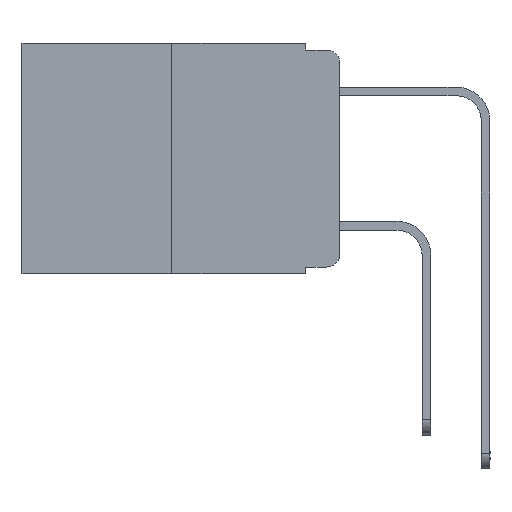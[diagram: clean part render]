
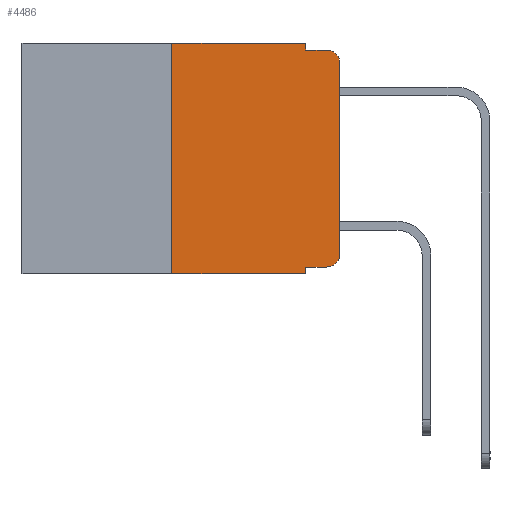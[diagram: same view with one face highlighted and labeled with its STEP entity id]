
A CAD part, left-side view. The second image highlights one B-rep face of the part: STEP entity #4486.
In plain terms, the highlighted planar face has unit normal (-1, 0, 0).
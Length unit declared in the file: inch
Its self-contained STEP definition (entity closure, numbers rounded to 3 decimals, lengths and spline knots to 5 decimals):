
#45 = DIRECTION ( 'NONE',  ( -1., 0., 0. ) ) ;
#456 = VERTEX_POINT ( 'NONE', #20318 ) ;
#701 = LINE ( 'NONE', #8829, #18971 ) ;
#1028 = VECTOR ( 'NONE', #3928, 39.37008 ) ;
#1140 = CARTESIAN_POINT ( 'NONE',  ( 0., 0.051, -0.01 ) ) ;
#1705 = DIRECTION ( 'NONE',  ( 0., 0., 1. ) ) ;
#2009 = VECTOR ( 'NONE', #10978, 39.37008 ) ;
#2176 = CARTESIAN_POINT ( 'NONE',  ( 0., 0.473, 0. ) ) ;
#2406 = LINE ( 'NONE', #10413, #20701 ) ;
#2830 = ORIENTED_EDGE ( 'NONE', *, *, #7244, .T. ) ;
#2980 = EDGE_CURVE ( 'NONE', #456, #15234, #11552, .T. ) ;
#3083 = CARTESIAN_POINT ( 'NONE',  ( 0., 0.02, -0.01 ) ) ;
#3471 = CARTESIAN_POINT ( 'NONE',  ( 0., 0.051, -0.01 ) ) ;
#3573 = CIRCLE ( 'NONE', #6258, 0.02 ) ;
#3658 = EDGE_CURVE ( 'NONE', #19618, #13431, #4326, .T. ) ;
#3928 = DIRECTION ( 'NONE',  ( 0., 0., -1. ) ) ;
#4113 = VECTOR ( 'NONE', #19249, 39.37008 ) ;
#4326 = LINE ( 'NONE', #6015, #2009 ) ;
#4486 = ADVANCED_FACE ( 'NONE', ( #10200 ), #16585, .F. ) ;
#4967 = DIRECTION ( 'NONE',  ( -1., 0., 0. ) ) ;
#5050 = DIRECTION ( 'NONE',  ( 0., -1., 0. ) ) ;
#5337 = EDGE_CURVE ( 'NONE', #8078, #17137, #15174, .T. ) ;
#5534 = CARTESIAN_POINT ( 'NONE',  ( 0., 0., -0.313 ) ) ;
#5756 = VECTOR ( 'NONE', #8558, 39.37008 ) ;
#6015 = CARTESIAN_POINT ( 'NONE',  ( 0., 0.051, 0. ) ) ;
#6071 = LINE ( 'NONE', #15951, #4113 ) ;
#6195 = EDGE_CURVE ( 'NONE', #8078, #17324, #6071, .T. ) ;
#6258 = AXIS2_PLACEMENT_3D ( 'NONE', #11697, #4967, #9713 ) ;
#6371 = CARTESIAN_POINT ( 'NONE',  ( 0., 0.473, -0.343 ) ) ;
#6826 = DIRECTION ( 'NONE',  ( 0., 0., 1. ) ) ;
#6879 = ORIENTED_EDGE ( 'NONE', *, *, #5337, .F. ) ;
#6883 = EDGE_CURVE ( 'NONE', #12221, #17137, #20797, .T. ) ;
#7235 = DIRECTION ( 'NONE',  ( 0., -1., 0. ) ) ;
#7244 = EDGE_CURVE ( 'NONE', #15883, #456, #13177, .T. ) ;
#7904 = VERTEX_POINT ( 'NONE', #17310 ) ;
#8078 = VERTEX_POINT ( 'NONE', #15833 ) ;
#8190 = CARTESIAN_POINT ( 'NONE',  ( 0., 0.02, -0.03 ) ) ;
#8558 = DIRECTION ( 'NONE',  ( 0., -1., 0. ) ) ;
#8595 = DIRECTION ( 'NONE',  ( 1., 0., 0. ) ) ;
#8617 = EDGE_LOOP ( 'NONE', ( #2830, #19640, #17640, #19344, #13300, #9917, #18479, #6879, #20110, #9728 ) ) ;
#8620 = CARTESIAN_POINT ( 'NONE',  ( 0., 0.051, 0. ) ) ;
#8829 = CARTESIAN_POINT ( 'NONE',  ( 0., 0.25, 0. ) ) ;
#9059 = EDGE_CURVE ( 'NONE', #12221, #7904, #701, .T. ) ;
#9549 = AXIS2_PLACEMENT_3D ( 'NONE', #8190, #45, #19259 ) ;
#9713 = DIRECTION ( 'NONE',  ( 0., 0., -1. ) ) ;
#9728 = ORIENTED_EDGE ( 'NONE', *, *, #16754, .T. ) ;
#9917 = ORIENTED_EDGE ( 'NONE', *, *, #9059, .F. ) ;
#10200 = FACE_OUTER_BOUND ( 'NONE', #8617, .T. ) ;
#10413 = CARTESIAN_POINT ( 'NONE',  ( 0., 0.473, 0. ) ) ;
#10791 = AXIS2_PLACEMENT_3D ( 'NONE', #2176, #8595, #15007 ) ;
#10978 = DIRECTION ( 'NONE',  ( 0., 0., -1. ) ) ;
#11257 = EDGE_CURVE ( 'NONE', #7904, #19618, #2406, .T. ) ;
#11552 = CIRCLE ( 'NONE', #9549, 0.02 ) ;
#11676 = LINE ( 'NONE', #3471, #17716 ) ;
#11697 = CARTESIAN_POINT ( 'NONE',  ( 0., 0.02, -0.313 ) ) ;
#11931 = CARTESIAN_POINT ( 'NONE',  ( 0., 0.051, 0. ) ) ;
#12221 = VERTEX_POINT ( 'NONE', #17248 ) ;
#13177 = LINE ( 'NONE', #14440, #16853 ) ;
#13300 = ORIENTED_EDGE ( 'NONE', *, *, #11257, .F. ) ;
#13431 = VERTEX_POINT ( 'NONE', #1140 ) ;
#13726 = EDGE_CURVE ( 'NONE', #13431, #15234, #11676, .T. ) ;
#14440 = CARTESIAN_POINT ( 'NONE',  ( 0., 0., 0. ) ) ;
#15007 = DIRECTION ( 'NONE',  ( 0., 0., -1. ) ) ;
#15174 = LINE ( 'NONE', #11931, #1028 ) ;
#15234 = VERTEX_POINT ( 'NONE', #3083 ) ;
#15833 = CARTESIAN_POINT ( 'NONE',  ( 0., 0.051, -0.333 ) ) ;
#15883 = VERTEX_POINT ( 'NONE', #5534 ) ;
#15951 = CARTESIAN_POINT ( 'NONE',  ( 0., 0.051, -0.333 ) ) ;
#16585 = PLANE ( 'NONE',  #10791 ) ;
#16754 = EDGE_CURVE ( 'NONE', #17324, #15883, #3573, .T. ) ;
#16853 = VECTOR ( 'NONE', #1705, 39.37008 ) ;
#17137 = VERTEX_POINT ( 'NONE', #19265 ) ;
#17248 = CARTESIAN_POINT ( 'NONE',  ( 0., 0.25, -0.343 ) ) ;
#17310 = CARTESIAN_POINT ( 'NONE',  ( 0., 0.25, 0. ) ) ;
#17324 = VERTEX_POINT ( 'NONE', #20095 ) ;
#17640 = ORIENTED_EDGE ( 'NONE', *, *, #13726, .F. ) ;
#17716 = VECTOR ( 'NONE', #5050, 39.37008 ) ;
#18479 = ORIENTED_EDGE ( 'NONE', *, *, #6883, .T. ) ;
#18971 = VECTOR ( 'NONE', #6826, 39.37008 ) ;
#19249 = DIRECTION ( 'NONE',  ( 0., -1., 0. ) ) ;
#19259 = DIRECTION ( 'NONE',  ( 0., 0., -1. ) ) ;
#19265 = CARTESIAN_POINT ( 'NONE',  ( 0., 0.051, -0.343 ) ) ;
#19344 = ORIENTED_EDGE ( 'NONE', *, *, #3658, .F. ) ;
#19618 = VERTEX_POINT ( 'NONE', #8620 ) ;
#19640 = ORIENTED_EDGE ( 'NONE', *, *, #2980, .T. ) ;
#20095 = CARTESIAN_POINT ( 'NONE',  ( 0., 0.02, -0.333 ) ) ;
#20110 = ORIENTED_EDGE ( 'NONE', *, *, #6195, .T. ) ;
#20318 = CARTESIAN_POINT ( 'NONE',  ( 0., 0., -0.03 ) ) ;
#20701 = VECTOR ( 'NONE', #7235, 39.37008 ) ;
#20797 = LINE ( 'NONE', #6371, #5756 ) ;
